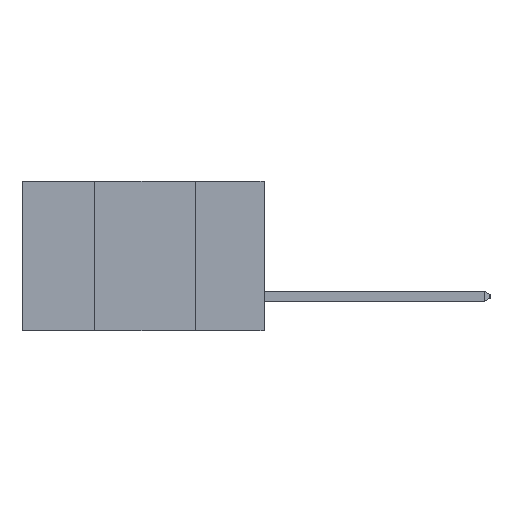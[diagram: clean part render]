
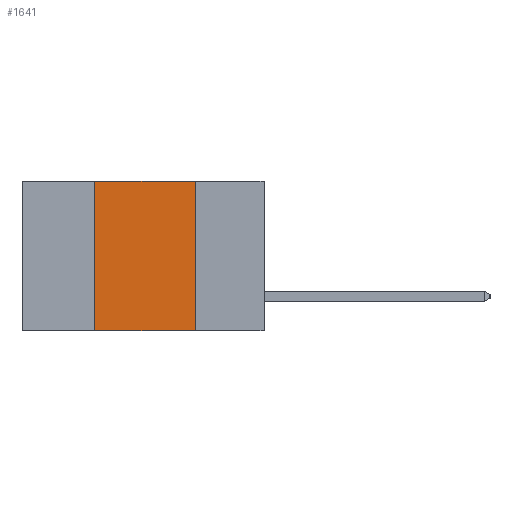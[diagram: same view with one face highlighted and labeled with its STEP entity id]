
A CAD part, left-side view. The second image highlights one B-rep face of the part: STEP entity #1641.
In plain terms, the highlighted planar face has unit normal (-1, 0, 0).
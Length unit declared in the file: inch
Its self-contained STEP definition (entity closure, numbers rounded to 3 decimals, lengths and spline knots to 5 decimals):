
#507 = CARTESIAN_POINT ( 'NONE',  ( 0., 0.6, 0. ) ) ;
#812 = LINE ( 'NONE', #507, #10281 ) ;
#1641 = ADVANCED_FACE ( 'NONE', ( #3118 ), #6247, .F. ) ;
#1705 = VERTEX_POINT ( 'NONE', #5795 ) ;
#2199 = CARTESIAN_POINT ( 'NONE',  ( 0., 0.17, -0.37 ) ) ;
#2423 = CARTESIAN_POINT ( 'NONE',  ( 0., 0.42, -0.37 ) ) ;
#2707 = VERTEX_POINT ( 'NONE', #10326 ) ;
#3118 = FACE_OUTER_BOUND ( 'NONE', #8271, .T. ) ;
#3182 = VERTEX_POINT ( 'NONE', #3267 ) ;
#3267 = CARTESIAN_POINT ( 'NONE',  ( 0., 0.17, 0. ) ) ;
#3955 = EDGE_CURVE ( 'NONE', #1705, #5130, #10760, .T. ) ;
#5130 = VERTEX_POINT ( 'NONE', #9201 ) ;
#5339 = EDGE_CURVE ( 'NONE', #3182, #2707, #10593, .T. ) ;
#5795 = CARTESIAN_POINT ( 'NONE',  ( 0., 0.42, -0.37 ) ) ;
#6035 = LINE ( 'NONE', #8597, #10258 ) ;
#6126 = VECTOR ( 'NONE', #9368, 39.37008 ) ;
#6163 = ORIENTED_EDGE ( 'NONE', *, *, #8422, .F. ) ;
#6179 = DIRECTION ( 'NONE',  ( 0., 0., -1. ) ) ;
#6196 = DIRECTION ( 'NONE',  ( 1., 0., 0. ) ) ;
#6207 = DIRECTION ( 'NONE',  ( 0., 0., 1. ) ) ;
#6247 = PLANE ( 'NONE',  #9360 ) ;
#6352 = CARTESIAN_POINT ( 'NONE',  ( 0., 0.6, 0. ) ) ;
#7754 = DIRECTION ( 'NONE',  ( 0., -1., 0. ) ) ;
#8271 = EDGE_LOOP ( 'NONE', ( #9673, #6163, #8423, #10632 ) ) ;
#8422 = EDGE_CURVE ( 'NONE', #5130, #3182, #812, .T. ) ;
#8423 = ORIENTED_EDGE ( 'NONE', *, *, #3955, .F. ) ;
#8547 = VECTOR ( 'NONE', #6207, 39.37008 ) ;
#8597 = CARTESIAN_POINT ( 'NONE',  ( 0., 0.6, -0.37 ) ) ;
#8964 = EDGE_CURVE ( 'NONE', #1705, #2707, #6035, .T. ) ;
#8983 = DIRECTION ( 'NONE',  ( 0., -1., 0. ) ) ;
#9201 = CARTESIAN_POINT ( 'NONE',  ( 0., 0.42, 0. ) ) ;
#9360 = AXIS2_PLACEMENT_3D ( 'NONE', #6352, #6196, #6179 ) ;
#9368 = DIRECTION ( 'NONE',  ( 0., 0., -1. ) ) ;
#9673 = ORIENTED_EDGE ( 'NONE', *, *, #5339, .F. ) ;
#10258 = VECTOR ( 'NONE', #7754, 39.37008 ) ;
#10281 = VECTOR ( 'NONE', #8983, 39.37008 ) ;
#10326 = CARTESIAN_POINT ( 'NONE',  ( 0., 0.17, -0.37 ) ) ;
#10593 = LINE ( 'NONE', #2199, #6126 ) ;
#10632 = ORIENTED_EDGE ( 'NONE', *, *, #8964, .T. ) ;
#10760 = LINE ( 'NONE', #2423, #8547 ) ;
